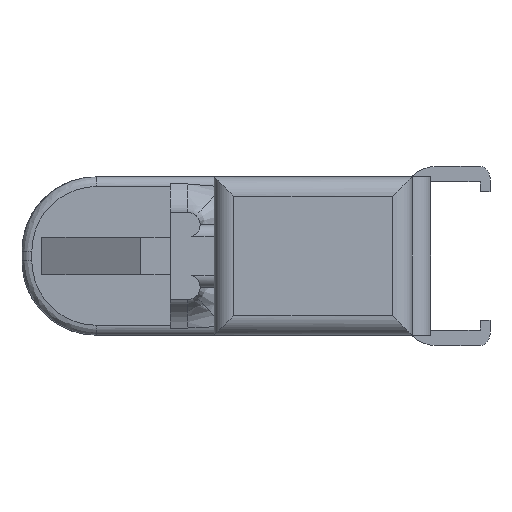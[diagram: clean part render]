
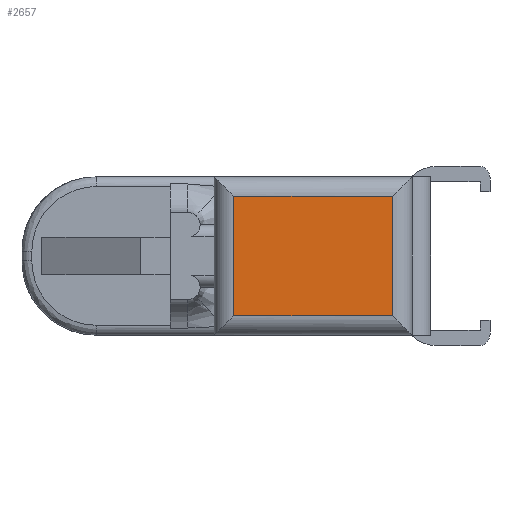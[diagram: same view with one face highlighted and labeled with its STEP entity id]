
A CAD part, front view. The second image highlights one B-rep face of the part: STEP entity #2657.
In plain terms, the highlighted planar face has unit normal (0, -1, 0).
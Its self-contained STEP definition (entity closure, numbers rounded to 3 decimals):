
#398 = DIRECTION ( 'NONE',  ( 1., 0., 0. ) ) ;
#449 = EDGE_CURVE ( 'NONE', #5920, #11502, #11948, .T. ) ;
#593 = CARTESIAN_POINT ( 'NONE',  ( 0., -35.56, 5. ) ) ;
#619 = CARTESIAN_POINT ( 'NONE',  ( -35.78, -35.56, 35.64 ) ) ;
#1502 = EDGE_CURVE ( 'NONE', #9752, #11502, #9566, .T. ) ;
#2377 = AXIS2_PLACEMENT_3D ( 'NONE', #2612, #10753, #3453 ) ;
#2612 = CARTESIAN_POINT ( 'NONE',  ( 0., -35.56, 0. ) ) ;
#2657 = ADVANCED_FACE ( 'NONE', ( #13251 ), #9744, .T. ) ;
#2691 = CARTESIAN_POINT ( 'NONE',  ( -76.58, -35.56, 5. ) ) ;
#3432 = CARTESIAN_POINT ( 'NONE',  ( 0., -35.56, 35.64 ) ) ;
#3453 = DIRECTION ( 'NONE',  ( 1., 0., 0. ) ) ;
#3729 = EDGE_CURVE ( 'NONE', #6415, #9752, #4777, .T. ) ;
#4034 = VECTOR ( 'NONE', #6734, 1000. ) ;
#4777 = LINE ( 'NONE', #3432, #5253 ) ;
#4795 = ORIENTED_EDGE ( 'NONE', *, *, #1502, .F. ) ;
#5054 = ORIENTED_EDGE ( 'NONE', *, *, #7310, .T. ) ;
#5253 = VECTOR ( 'NONE', #398, 1000. ) ;
#5488 = LINE ( 'NONE', #7741, #4034 ) ;
#5920 = VERTEX_POINT ( 'NONE', #2691 ) ;
#6415 = VERTEX_POINT ( 'NONE', #10869 ) ;
#6722 = VECTOR ( 'NONE', #8204, 1000. ) ;
#6734 = DIRECTION ( 'NONE',  ( 0., 0., -1. ) ) ;
#6850 = ORIENTED_EDGE ( 'NONE', *, *, #3729, .F. ) ;
#7310 = EDGE_CURVE ( 'NONE', #6415, #5920, #5488, .T. ) ;
#7741 = CARTESIAN_POINT ( 'NONE',  ( -76.58, -35.56, 0. ) ) ;
#8204 = DIRECTION ( 'NONE',  ( 1., 0., 0. ) ) ;
#8251 = VECTOR ( 'NONE', #13399, 1000. ) ;
#9122 = CARTESIAN_POINT ( 'NONE',  ( -35.78, -35.56, 0. ) ) ;
#9566 = LINE ( 'NONE', #9122, #8251 ) ;
#9744 = PLANE ( 'NONE',  #2377 ) ;
#9752 = VERTEX_POINT ( 'NONE', #619 ) ;
#10753 = DIRECTION ( 'NONE',  ( 0., -1., 0. ) ) ;
#10869 = CARTESIAN_POINT ( 'NONE',  ( -76.58, -35.56, 35.64 ) ) ;
#11245 = CARTESIAN_POINT ( 'NONE',  ( -35.78, -35.56, 5. ) ) ;
#11502 = VERTEX_POINT ( 'NONE', #11245 ) ;
#11725 = ORIENTED_EDGE ( 'NONE', *, *, #449, .T. ) ;
#11948 = LINE ( 'NONE', #593, #6722 ) ;
#13095 = EDGE_LOOP ( 'NONE', ( #4795, #6850, #5054, #11725 ) ) ;
#13251 = FACE_OUTER_BOUND ( 'NONE', #13095, .T. ) ;
#13399 = DIRECTION ( 'NONE',  ( 0., 0., -1. ) ) ;
